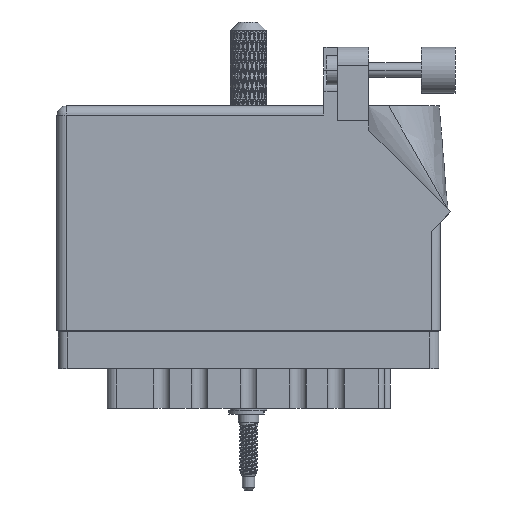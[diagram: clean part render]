
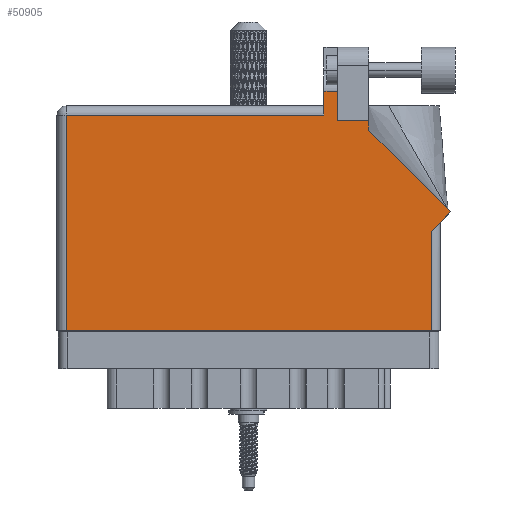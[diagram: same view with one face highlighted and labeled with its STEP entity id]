
A CAD part, front view. The second image highlights one B-rep face of the part: STEP entity #50905.
In plain terms, the highlighted face is planar.
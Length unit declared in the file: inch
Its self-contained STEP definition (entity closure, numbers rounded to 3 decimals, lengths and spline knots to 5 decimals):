
#1763 = VERTEX_POINT ( 'NONE', #8141 ) ;
#2701 = LINE ( 'NONE', #36555, #79253 ) ;
#3374 = ORIENTED_EDGE ( 'NONE', *, *, #98857, .T. ) ;
#3800 = VERTEX_POINT ( 'NONE', #77716 ) ;
#4235 = ORIENTED_EDGE ( 'NONE', *, *, #20253, .T. ) ;
#4454 = VERTEX_POINT ( 'NONE', #69391 ) ;
#5290 = CARTESIAN_POINT ( 'NONE',  ( 0., 1.53, 0. ) ) ;
#5491 = ORIENTED_EDGE ( 'NONE', *, *, #101117, .T. ) ;
#8141 = CARTESIAN_POINT ( 'NONE',  ( 0.062, 0., 0. ) ) ;
#9540 = VERTEX_POINT ( 'NONE', #88081 ) ;
#12485 = EDGE_CURVE ( 'NONE', #116393, #3800, #39026, .T. ) ;
#14606 = CARTESIAN_POINT ( 'NONE',  ( 1.819, 1.53, 0. ) ) ;
#15786 = CARTESIAN_POINT ( 'NONE',  ( 2.68271, 0.80771, 0. ) ) ;
#16133 = CARTESIAN_POINT ( 'NONE',  ( 2.55, 0., 0. ) ) ;
#17537 = LINE ( 'NONE', #14606, #24665 ) ;
#20253 = EDGE_CURVE ( 'NONE', #76217, #87306, #106332, .T. ) ;
#21267 = EDGE_CURVE ( 'NONE', #1763, #107260, #91558, .T. ) ;
#22634 = VECTOR ( 'NONE', #70033, 39.37008 ) ;
#24275 = DIRECTION ( 'NONE',  ( 0., -1., 0. ) ) ;
#24665 = VECTOR ( 'NONE', #70673, 39.37008 ) ;
#25309 = ORIENTED_EDGE ( 'NONE', *, *, #118363, .T. ) ;
#26382 = CARTESIAN_POINT ( 'NONE',  ( 0., 1.468, 0. ) ) ;
#29140 = ORIENTED_EDGE ( 'NONE', *, *, #31142, .T. ) ;
#30543 = ORIENTED_EDGE ( 'NONE', *, *, #73445, .T. ) ;
#30634 = ORIENTED_EDGE ( 'NONE', *, *, #21267, .T. ) ;
#31142 = EDGE_CURVE ( 'NONE', #87306, #9540, #17537, .T. ) ;
#34084 = VECTOR ( 'NONE', #24275, 39.37008 ) ;
#36555 = CARTESIAN_POINT ( 'NONE',  ( 2.126, 1.43, 0. ) ) ;
#39026 = LINE ( 'NONE', #39141, #49078 ) ;
#39141 = CARTESIAN_POINT ( 'NONE',  ( 2.68271, 0.80771, 0. ) ) ;
#40958 = VECTOR ( 'NONE', #108704, 39.37008 ) ;
#41283 = LINE ( 'NONE', #116695, #34084 ) ;
#41717 = EDGE_LOOP ( 'NONE', ( #5491, #4235, #29140, #3374, #114725, #30634, #25309, #42179, #111358, #30543, #52697 ) ) ;
#42179 = ORIENTED_EDGE ( 'NONE', *, *, #81701, .T. ) ;
#47523 = DIRECTION ( 'NONE',  ( 0., 1., 0. ) ) ;
#49078 = VECTOR ( 'NONE', #56470, 39.37008 ) ;
#49654 = CARTESIAN_POINT ( 'NONE',  ( 1.819, 1.6315, 0. ) ) ;
#50905 = ADVANCED_FACE ( 'NONE', ( #112197 ), #61398, .F. ) ;
#52660 = VERTEX_POINT ( 'NONE', #87414 ) ;
#52697 = ORIENTED_EDGE ( 'NONE', *, *, #115648, .T. ) ;
#52799 = VECTOR ( 'NONE', #97277, 39.37008 ) ;
#53931 = DIRECTION ( 'NONE',  ( -1., 0., 0. ) ) ;
#56470 = DIRECTION ( 'NONE',  ( -0.707, 0.707, 0. ) ) ;
#59239 = DIRECTION ( 'NONE',  ( 0.707, 0.707, 0. ) ) ;
#59921 = VECTOR ( 'NONE', #108471, 39.37008 ) ;
#61009 = DIRECTION ( 'NONE',  ( 0., 0., -1. ) ) ;
#61398 = PLANE ( 'NONE',  #110018 ) ;
#62374 = VECTOR ( 'NONE', #47523, 39.37008 ) ;
#66587 = VECTOR ( 'NONE', #113652, 39.37008 ) ;
#67062 = LINE ( 'NONE', #99706, #52799 ) ;
#69391 = CARTESIAN_POINT ( 'NONE',  ( 0.062, 1.468, 0. ) ) ;
#69466 = DIRECTION ( 'NONE',  ( -1., 0., 0. ) ) ;
#69712 = CARTESIAN_POINT ( 'NONE',  ( 2.612, 0.737, 0. ) ) ;
#70033 = DIRECTION ( 'NONE',  ( -1., 0., 0. ) ) ;
#70673 = DIRECTION ( 'NONE',  ( 0., -1., 0. ) ) ;
#70857 = VERTEX_POINT ( 'NONE', #83285 ) ;
#72737 = LINE ( 'NONE', #69712, #100131 ) ;
#73445 = EDGE_CURVE ( 'NONE', #3800, #52660, #118695, .T. ) ;
#76217 = VERTEX_POINT ( 'NONE', #81493 ) ;
#77716 = CARTESIAN_POINT ( 'NONE',  ( 2.126, 1.36442, 0. ) ) ;
#79253 = VECTOR ( 'NONE', #53931, 39.37008 ) ;
#81493 = CARTESIAN_POINT ( 'NONE',  ( 1.913, 1.6315, 0. ) ) ;
#81701 = EDGE_CURVE ( 'NONE', #108135, #116393, #72737, .T. ) ;
#83285 = CARTESIAN_POINT ( 'NONE',  ( 1.913, 1.43, 0. ) ) ;
#87306 = VERTEX_POINT ( 'NONE', #49654 ) ;
#87414 = CARTESIAN_POINT ( 'NONE',  ( 2.126, 1.43, 0. ) ) ;
#88081 = CARTESIAN_POINT ( 'NONE',  ( 1.819, 1.468, 0. ) ) ;
#91558 = LINE ( 'NONE', #117004, #59921 ) ;
#93040 = CARTESIAN_POINT ( 'NONE',  ( 2.126, 1.36442, 0. ) ) ;
#95044 = CARTESIAN_POINT ( 'NONE',  ( 1.913, 1.43, 0. ) ) ;
#95670 = EDGE_CURVE ( 'NONE', #4454, #1763, #41283, .T. ) ;
#97277 = DIRECTION ( 'NONE',  ( 0., 1., 0. ) ) ;
#98857 = EDGE_CURVE ( 'NONE', #9540, #4454, #116102, .T. ) ;
#99706 = CARTESIAN_POINT ( 'NONE',  ( 2.55, 0.737, 0. ) ) ;
#100131 = VECTOR ( 'NONE', #59239, 39.37008 ) ;
#100881 = CARTESIAN_POINT ( 'NONE',  ( 2.55, 0.675, 0. ) ) ;
#101117 = EDGE_CURVE ( 'NONE', #70857, #76217, #109934, .T. ) ;
#106332 = LINE ( 'NONE', #106364, #22634 ) ;
#106364 = CARTESIAN_POINT ( 'NONE',  ( 2.24377, 1.6315, 0. ) ) ;
#107260 = VERTEX_POINT ( 'NONE', #16133 ) ;
#108135 = VERTEX_POINT ( 'NONE', #100881 ) ;
#108471 = DIRECTION ( 'NONE',  ( 1., 0., 0. ) ) ;
#108704 = DIRECTION ( 'NONE',  ( -1., 0., 0. ) ) ;
#109934 = LINE ( 'NONE', #95044, #66587 ) ;
#110018 = AXIS2_PLACEMENT_3D ( 'NONE', #5290, #61009, #69466 ) ;
#111358 = ORIENTED_EDGE ( 'NONE', *, *, #12485, .T. ) ;
#112197 = FACE_OUTER_BOUND ( 'NONE', #41717, .T. ) ;
#113652 = DIRECTION ( 'NONE',  ( 0., 1., 0. ) ) ;
#114725 = ORIENTED_EDGE ( 'NONE', *, *, #95670, .T. ) ;
#115648 = EDGE_CURVE ( 'NONE', #52660, #70857, #2701, .T. ) ;
#116102 = LINE ( 'NONE', #26382, #40958 ) ;
#116393 = VERTEX_POINT ( 'NONE', #15786 ) ;
#116695 = CARTESIAN_POINT ( 'NONE',  ( 0.062, 0., 0. ) ) ;
#117004 = CARTESIAN_POINT ( 'NONE',  ( 0., 0., 0. ) ) ;
#118363 = EDGE_CURVE ( 'NONE', #107260, #108135, #67062, .T. ) ;
#118695 = LINE ( 'NONE', #93040, #62374 ) ;
